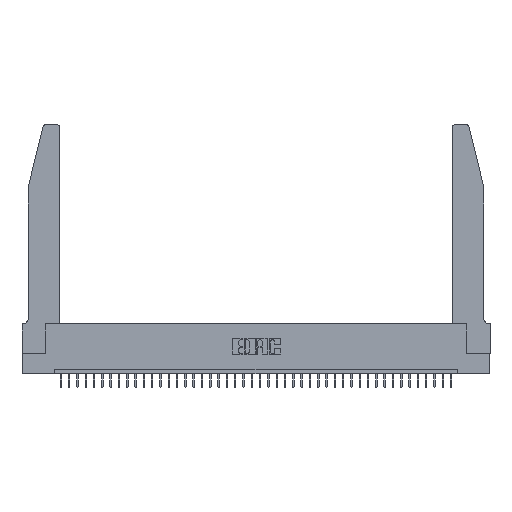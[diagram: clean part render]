
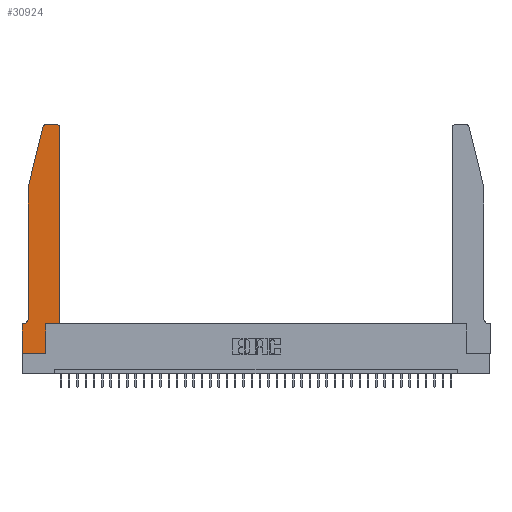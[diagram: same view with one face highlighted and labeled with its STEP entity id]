
A CAD part, top view. The second image highlights one B-rep face of the part: STEP entity #30924.
In plain terms, the highlighted planar face has unit normal (0, 0, 1).
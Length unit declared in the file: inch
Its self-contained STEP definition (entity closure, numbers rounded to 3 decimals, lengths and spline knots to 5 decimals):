
#842 = CARTESIAN_POINT ( 'NONE',  ( 0.0755, 2., 0.37 ) ) ;
#1040 = VERTEX_POINT ( 'NONE', #20063 ) ;
#1106 = DIRECTION ( 'NONE',  ( 0., 1., 0. ) ) ;
#1135 = LINE ( 'NONE', #35591, #32132 ) ;
#1234 = CARTESIAN_POINT ( 'NONE',  ( 0.4505, 0.35, 0.37 ) ) ;
#2103 = CARTESIAN_POINT ( 'NONE',  ( 0.284, 2.72, 0.37 ) ) ;
#2154 = DIRECTION ( 'NONE',  ( 1., 0., 0. ) ) ;
#3146 = CARTESIAN_POINT ( 'NONE',  ( 0.4505, 2.72, 0.37 ) ) ;
#3723 = DIRECTION ( 'NONE',  ( -1., 0., 0. ) ) ;
#3822 = LINE ( 'NONE', #19907, #31885 ) ;
#3836 = VERTEX_POINT ( 'NONE', #34971 ) ;
#3848 = AXIS2_PLACEMENT_3D ( 'NONE', #12261, #36800, #11997 ) ;
#5210 = LINE ( 'NONE', #29424, #6179 ) ;
#5555 = VERTEX_POINT ( 'NONE', #26416 ) ;
#5664 = LINE ( 'NONE', #18101, #39639 ) ;
#6179 = VECTOR ( 'NONE', #11323, 39.37008 ) ;
#7018 = CARTESIAN_POINT ( 'NONE',  ( 0.2865, 0.35, 0.37 ) ) ;
#7021 = ORIENTED_EDGE ( 'NONE', *, *, #16536, .T. ) ;
#7359 = CIRCLE ( 'NONE', #13798, 0.03 ) ;
#8322 = EDGE_CURVE ( 'NONE', #35729, #11666, #3822, .T. ) ;
#8516 = CARTESIAN_POINT ( 'NONE',  ( 0.4205, 2.72, 0.37 ) ) ;
#9766 = VECTOR ( 'NONE', #1106, 39.37008 ) ;
#10592 = ORIENTED_EDGE ( 'NONE', *, *, #10685, .T. ) ;
#10685 = EDGE_CURVE ( 'NONE', #30388, #38369, #26856, .T. ) ;
#10968 = LINE ( 'NONE', #842, #25469 ) ;
#11323 = DIRECTION ( 'NONE',  ( -1., 0., 0. ) ) ;
#11475 = EDGE_CURVE ( 'NONE', #28709, #27239, #1135, .T. ) ;
#11666 = VERTEX_POINT ( 'NONE', #38100 ) ;
#11914 = DIRECTION ( 'NONE',  ( 0., 0., 1. ) ) ;
#11997 = DIRECTION ( 'NONE',  ( -1., 0., 0. ) ) ;
#12261 = CARTESIAN_POINT ( 'NONE',  ( 0.0055, 0.42, 0.37 ) ) ;
#12380 = CARTESIAN_POINT ( 'NONE',  ( 0.4505, 0.35, 0.37 ) ) ;
#12530 = CARTESIAN_POINT ( 'NONE',  ( 0.284, 2.75, 0.37 ) ) ;
#13284 = VECTOR ( 'NONE', #3723, 39.37008 ) ;
#13428 = DIRECTION ( 'NONE',  ( 0., -1., 0. ) ) ;
#13600 = LINE ( 'NONE', #25122, #20854 ) ;
#13798 = AXIS2_PLACEMENT_3D ( 'NONE', #8516, #11914, #2154 ) ;
#14354 = VERTEX_POINT ( 'NONE', #30695 ) ;
#15444 = DIRECTION ( 'NONE',  ( 1., 0., 0. ) ) ;
#15526 = CIRCLE ( 'NONE', #3848, 0.07 ) ;
#16536 = EDGE_CURVE ( 'NONE', #27239, #40101, #21358, .T. ) ;
#17507 = AXIS2_PLACEMENT_3D ( 'NONE', #2103, #26337, #29419 ) ;
#17788 = AXIS2_PLACEMENT_3D ( 'NONE', #36765, #39903, #15444 ) ;
#18101 = CARTESIAN_POINT ( 'NONE',  ( 0., 0., 0.37 ) ) ;
#18649 = CARTESIAN_POINT ( 'NONE',  ( 0.0755, 2., 0.37 ) ) ;
#19907 = CARTESIAN_POINT ( 'NONE',  ( 0., 0., 0.37 ) ) ;
#20063 = CARTESIAN_POINT ( 'NONE',  ( 0.0055, 0.35, 0.37 ) ) ;
#20385 = ORIENTED_EDGE ( 'NONE', *, *, #8322, .T. ) ;
#20854 = VECTOR ( 'NONE', #21969, 39.37008 ) ;
#21163 = VECTOR ( 'NONE', #25243, 39.37008 ) ;
#21358 = LINE ( 'NONE', #1234, #9766 ) ;
#21402 = ORIENTED_EDGE ( 'NONE', *, *, #24257, .T. ) ;
#21969 = DIRECTION ( 'NONE',  ( -0.239, -0.971, 0. ) ) ;
#22240 = CARTESIAN_POINT ( 'NONE',  ( 0.2605, 2.75, 0.37 ) ) ;
#22694 = CARTESIAN_POINT ( 'NONE',  ( 0., 0., 0.37 ) ) ;
#23110 = EDGE_LOOP ( 'NONE', ( #10592, #34104, #28870, #29410, #29364, #21402, #26327, #20385, #30081, #37617, #7021, #39951 ) ) ;
#24257 = EDGE_CURVE ( 'NONE', #1040, #14354, #5210, .T. ) ;
#25122 = CARTESIAN_POINT ( 'NONE',  ( 0.0755, 2., 0.37 ) ) ;
#25243 = DIRECTION ( 'NONE',  ( 0., 1., 0. ) ) ;
#25469 = VECTOR ( 'NONE', #13428, 39.37008 ) ;
#26327 = ORIENTED_EDGE ( 'NONE', *, *, #36586, .T. ) ;
#26337 = DIRECTION ( 'NONE',  ( 0., 0., 1. ) ) ;
#26416 = CARTESIAN_POINT ( 'NONE',  ( 0.25487, 2.72718, 0.37 ) ) ;
#26502 = DIRECTION ( 'NONE',  ( 1., 0., 0. ) ) ;
#26849 = EDGE_CURVE ( 'NONE', #11666, #28709, #29395, .T. ) ;
#26856 = LINE ( 'NONE', #22240, #13284 ) ;
#27239 = VERTEX_POINT ( 'NONE', #12380 ) ;
#27384 = EDGE_CURVE ( 'NONE', #36066, #3836, #10968, .T. ) ;
#27532 = FACE_OUTER_BOUND ( 'NONE', #23110, .T. ) ;
#28709 = VERTEX_POINT ( 'NONE', #7018 ) ;
#28870 = ORIENTED_EDGE ( 'NONE', *, *, #39556, .T. ) ;
#29236 = DIRECTION ( 'NONE',  ( 1., 0., 0. ) ) ;
#29364 = ORIENTED_EDGE ( 'NONE', *, *, #34655, .T. ) ;
#29395 = LINE ( 'NONE', #37344, #21163 ) ;
#29410 = ORIENTED_EDGE ( 'NONE', *, *, #27384, .T. ) ;
#29419 = DIRECTION ( 'NONE',  ( 1., 0., 0. ) ) ;
#29424 = CARTESIAN_POINT ( 'NONE',  ( 0.0755, 0.35, 0.37 ) ) ;
#29511 = EDGE_CURVE ( 'NONE', #38369, #5555, #30560, .T. ) ;
#30081 = ORIENTED_EDGE ( 'NONE', *, *, #26849, .T. ) ;
#30388 = VERTEX_POINT ( 'NONE', #36004 ) ;
#30560 = CIRCLE ( 'NONE', #17507, 0.03 ) ;
#30695 = CARTESIAN_POINT ( 'NONE',  ( 0., 0.35, 0.37 ) ) ;
#30924 = ADVANCED_FACE ( 'NONE', ( #27532 ), #39768, .T. ) ;
#31885 = VECTOR ( 'NONE', #29236, 39.37008 ) ;
#32132 = VECTOR ( 'NONE', #26502, 39.37008 ) ;
#34104 = ORIENTED_EDGE ( 'NONE', *, *, #29511, .T. ) ;
#34655 = EDGE_CURVE ( 'NONE', #3836, #1040, #15526, .T. ) ;
#34971 = CARTESIAN_POINT ( 'NONE',  ( 0.0755, 0.42, 0.37 ) ) ;
#35591 = CARTESIAN_POINT ( 'NONE',  ( 0.4505, 0.35, 0.37 ) ) ;
#35729 = VERTEX_POINT ( 'NONE', #22694 ) ;
#36004 = CARTESIAN_POINT ( 'NONE',  ( 0.4205, 2.75, 0.37 ) ) ;
#36066 = VERTEX_POINT ( 'NONE', #18649 ) ;
#36428 = DIRECTION ( 'NONE',  ( 0., -1., 0. ) ) ;
#36586 = EDGE_CURVE ( 'NONE', #14354, #35729, #5664, .T. ) ;
#36765 = CARTESIAN_POINT ( 'NONE',  ( 0., 0.35, 0.37 ) ) ;
#36800 = DIRECTION ( 'NONE',  ( 0., 0., -1. ) ) ;
#37344 = CARTESIAN_POINT ( 'NONE',  ( 0.2865, 0.35, 0.37 ) ) ;
#37617 = ORIENTED_EDGE ( 'NONE', *, *, #11475, .T. ) ;
#38100 = CARTESIAN_POINT ( 'NONE',  ( 0.2865, 0., 0.37 ) ) ;
#38369 = VERTEX_POINT ( 'NONE', #12530 ) ;
#39274 = EDGE_CURVE ( 'NONE', #40101, #30388, #7359, .T. ) ;
#39556 = EDGE_CURVE ( 'NONE', #5555, #36066, #13600, .T. ) ;
#39639 = VECTOR ( 'NONE', #36428, 39.37008 ) ;
#39768 = PLANE ( 'NONE',  #17788 ) ;
#39903 = DIRECTION ( 'NONE',  ( 0., 0., 1. ) ) ;
#39951 = ORIENTED_EDGE ( 'NONE', *, *, #39274, .T. ) ;
#40101 = VERTEX_POINT ( 'NONE', #3146 ) ;
